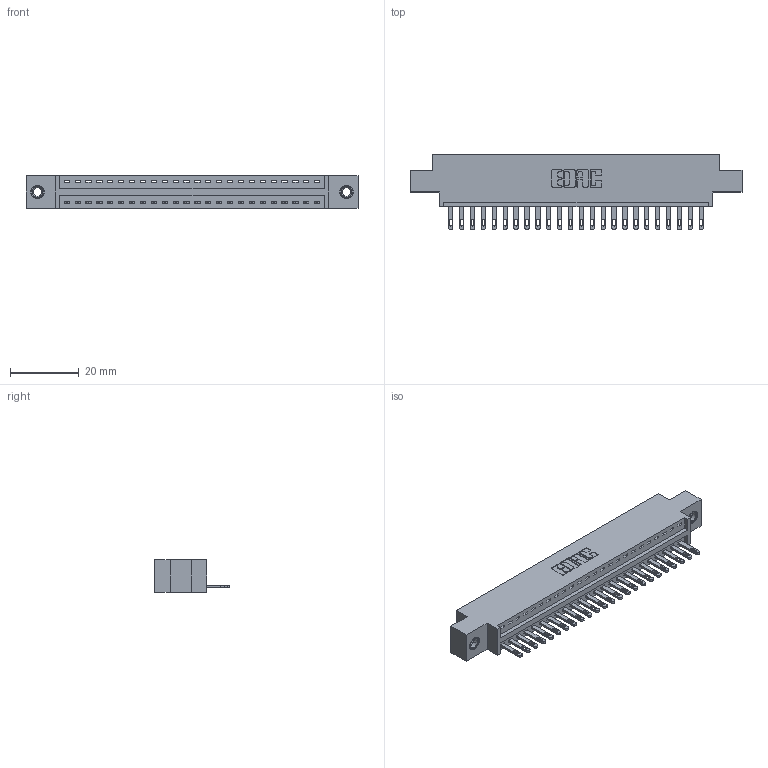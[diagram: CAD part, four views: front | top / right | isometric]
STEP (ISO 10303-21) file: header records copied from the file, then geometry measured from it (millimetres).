
FILE_DESCRIPTION (( 'STEP AP203' ), '1' );
FILE_NAME ('896-024-500-607.STEP', '2021-07-27T17:30:53', ( '' ), ( '' ), 'SwSTEP 2.0', 'SolidWorks 2020', '' );
FILE_SCHEMA (( 'CONFIG_CONTROL_DESIGN' ));
Length unit declared in the file: inch
Products named in the file (4): 846 Part_0.170 Offset - 0.156 Dia-TI; 345-292-001_345-293-100; 345-250-001_345-250-005-103; 896-024-500-607
Assembly tree (27 placements, depth 2):
  896-024-500-607
    846 Part_0.170 Offset - 0.156 Dia-TI
    345-292-001_345-293-100  x24
    345-250-001_345-250-005-103  x2
Bounding box: 96.77 x 21.84 x 9.4 mm (x, y, z)
Volume: 8986.1 mm3; surface area: 11288.2 mm2
Topology: 27 solids, 27 shells, 1482 faces, 4509 edges, 2998 vertices
Faces by surface type: plane 928, cylinder 538, cone 12, torus 4
Entity records: 18566 total; most frequent: CARTESIAN_POINT 3171, ORIENTED_EDGE 3122, DIRECTION 2847, EDGE_CURVE 1561, VECTOR 1309, LINE 1309, VERTEX_POINT 1036, AXIS2_PLACEMENT_3D 769
